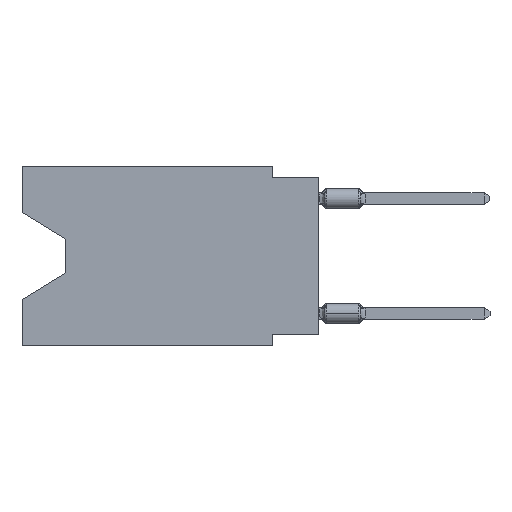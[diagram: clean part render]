
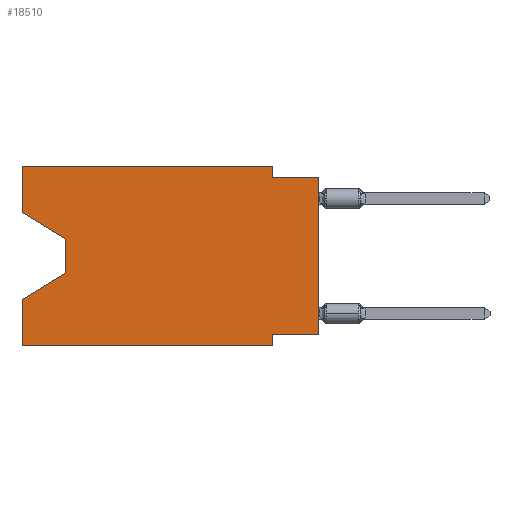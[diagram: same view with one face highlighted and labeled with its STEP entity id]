
A CAD part, left-side view. The second image highlights one B-rep face of the part: STEP entity #18510.
In plain terms, the highlighted planar face has unit normal (-1, 0, 0).
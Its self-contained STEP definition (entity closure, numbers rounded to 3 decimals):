
#665 = CARTESIAN_POINT ( 'NONE',  ( 0., 0., -0.635 ) ) ;
#674 = ORIENTED_EDGE ( 'NONE', *, *, #3548, .T. ) ;
#728 = LINE ( 'NONE', #2811, #1620 ) ;
#1167 = DIRECTION ( 'NONE',  ( 1., 0., 0. ) ) ;
#1458 = CARTESIAN_POINT ( 'NONE',  ( 0., 2.54, 0. ) ) ;
#1486 = ORIENTED_EDGE ( 'NONE', *, *, #24072, .F. ) ;
#1516 = VERTEX_POINT ( 'NONE', #9213 ) ;
#1619 = VERTEX_POINT ( 'NONE', #9345 ) ;
#1620 = VECTOR ( 'NONE', #18370, 1000. ) ;
#1637 = VERTEX_POINT ( 'NONE', #12419 ) ;
#2066 = VERTEX_POINT ( 'NONE', #665 ) ;
#2216 = VECTOR ( 'NONE', #14142, 1000. ) ;
#2474 = CARTESIAN_POINT ( 'NONE',  ( 0., 16.383, 0. ) ) ;
#2606 = VECTOR ( 'NONE', #7746, 1000. ) ;
#2622 = EDGE_CURVE ( 'NONE', #1619, #23544, #16702, .T. ) ;
#2811 = CARTESIAN_POINT ( 'NONE',  ( 0., 16.383, 0. ) ) ;
#2982 = AXIS2_PLACEMENT_3D ( 'NONE', #18926, #1167, #19428 ) ;
#3032 = VERTEX_POINT ( 'NONE', #24929 ) ;
#3123 = PLANE ( 'NONE',  #2982 ) ;
#3548 = EDGE_CURVE ( 'NONE', #1637, #2066, #16508, .T. ) ;
#4937 = CARTESIAN_POINT ( 'NONE',  ( 0., 16.383, -7.36 ) ) ;
#5001 = VECTOR ( 'NONE', #16237, 1000. ) ;
#5008 = VERTEX_POINT ( 'NONE', #15587 ) ;
#5181 = EDGE_CURVE ( 'NONE', #18726, #2066, #6169, .T. ) ;
#5586 = EDGE_LOOP ( 'NONE', ( #17032, #24458, #7455, #25322, #24687, #18570, #10149, #674, #22332, #18632, #1486, #10374 ) ) ;
#5853 = CARTESIAN_POINT ( 'NONE',  ( 0., 2.54, 0. ) ) ;
#5916 = VECTOR ( 'NONE', #11284, 1000. ) ;
#5964 = VECTOR ( 'NONE', #10813, 1000. ) ;
#5990 = DIRECTION ( 'NONE',  ( 0., 0., -1. ) ) ;
#6055 = LINE ( 'NONE', #19493, #2606 ) ;
#6169 = LINE ( 'NONE', #15846, #5001 ) ;
#6363 = VECTOR ( 'NONE', #22815, 1000. ) ;
#7059 = LINE ( 'NONE', #24748, #5964 ) ;
#7455 = ORIENTED_EDGE ( 'NONE', *, *, #19430, .T. ) ;
#7746 = DIRECTION ( 'NONE',  ( 0., -0.855, -0.519 ) ) ;
#8578 = EDGE_CURVE ( 'NONE', #25032, #18726, #14258, .T. ) ;
#8961 = CARTESIAN_POINT ( 'NONE',  ( 0., 16.383, 0. ) ) ;
#9213 = CARTESIAN_POINT ( 'NONE',  ( 0., 13.97, -5.893 ) ) ;
#9345 = CARTESIAN_POINT ( 'NONE',  ( 0., 16.383, -2.546 ) ) ;
#9884 = CARTESIAN_POINT ( 'NONE',  ( 0., 2.54, -0.635 ) ) ;
#9913 = CARTESIAN_POINT ( 'NONE',  ( 0., 13.97, -5.893 ) ) ;
#10149 = ORIENTED_EDGE ( 'NONE', *, *, #13811, .F. ) ;
#10374 = ORIENTED_EDGE ( 'NONE', *, *, #2622, .F. ) ;
#10813 = DIRECTION ( 'NONE',  ( 0., -1., 0. ) ) ;
#11152 = VECTOR ( 'NONE', #5990, 1000. ) ;
#11284 = DIRECTION ( 'NONE',  ( 0., 0., 1. ) ) ;
#11548 = VERTEX_POINT ( 'NONE', #15774 ) ;
#12119 = CARTESIAN_POINT ( 'NONE',  ( 0., 16.383, 0. ) ) ;
#12419 = CARTESIAN_POINT ( 'NONE',  ( 0., 0., -9.271 ) ) ;
#13000 = VECTOR ( 'NONE', #24486, 1000. ) ;
#13389 = VECTOR ( 'NONE', #21530, 1000. ) ;
#13648 = DIRECTION ( 'NONE',  ( 0., 0.855, -0.519 ) ) ;
#13811 = EDGE_CURVE ( 'NONE', #1637, #11548, #25047, .T. ) ;
#14142 = DIRECTION ( 'NONE',  ( 0., -1., 0. ) ) ;
#14258 = LINE ( 'NONE', #5853, #11152 ) ;
#14297 = LINE ( 'NONE', #22184, #13000 ) ;
#14510 = VERTEX_POINT ( 'NONE', #4937 ) ;
#14960 = DIRECTION ( 'NONE',  ( 0., 1., 0. ) ) ;
#15017 = VECTOR ( 'NONE', #13648, 1000. ) ;
#15587 = CARTESIAN_POINT ( 'NONE',  ( 0., 13.97, -4.013 ) ) ;
#15774 = CARTESIAN_POINT ( 'NONE',  ( 0., 2.54, -9.271 ) ) ;
#15846 = CARTESIAN_POINT ( 'NONE',  ( 0., 0., -0.635 ) ) ;
#16237 = DIRECTION ( 'NONE',  ( 0., -1., 0. ) ) ;
#16508 = LINE ( 'NONE', #24896, #13389 ) ;
#16702 = LINE ( 'NONE', #8961, #5916 ) ;
#17032 = ORIENTED_EDGE ( 'NONE', *, *, #18996, .T. ) ;
#17125 = VECTOR ( 'NONE', #14960, 1000. ) ;
#17431 = EDGE_CURVE ( 'NONE', #24689, #14510, #728, .T. ) ;
#17666 = LINE ( 'NONE', #9913, #15017 ) ;
#18370 = DIRECTION ( 'NONE',  ( 0., 0., 1. ) ) ;
#18413 = LINE ( 'NONE', #2474, #2216 ) ;
#18510 = ADVANCED_FACE ( 'NONE', ( #20850 ), #3123, .F. ) ;
#18570 = ORIENTED_EDGE ( 'NONE', *, *, #22584, .F. ) ;
#18632 = ORIENTED_EDGE ( 'NONE', *, *, #8578, .F. ) ;
#18726 = VERTEX_POINT ( 'NONE', #9884 ) ;
#18926 = CARTESIAN_POINT ( 'NONE',  ( 0., 16.383, 0. ) ) ;
#18996 = EDGE_CURVE ( 'NONE', #1619, #5008, #6055, .T. ) ;
#19209 = CARTESIAN_POINT ( 'NONE',  ( 0., 13.97, -4.013 ) ) ;
#19428 = DIRECTION ( 'NONE',  ( 0., 0., -1. ) ) ;
#19430 = EDGE_CURVE ( 'NONE', #1516, #14510, #17666, .T. ) ;
#19493 = CARTESIAN_POINT ( 'NONE',  ( 0., 16.383, -2.546 ) ) ;
#20850 = FACE_OUTER_BOUND ( 'NONE', #5586, .T. ) ;
#21530 = DIRECTION ( 'NONE',  ( 0., 0., 1. ) ) ;
#22184 = CARTESIAN_POINT ( 'NONE',  ( 0., 2.54, -9.906 ) ) ;
#22332 = ORIENTED_EDGE ( 'NONE', *, *, #5181, .F. ) ;
#22584 = EDGE_CURVE ( 'NONE', #11548, #3032, #14297, .T. ) ;
#22609 = EDGE_CURVE ( 'NONE', #24689, #3032, #7059, .T. ) ;
#22707 = CARTESIAN_POINT ( 'NONE',  ( 0., 0., -9.271 ) ) ;
#22815 = DIRECTION ( 'NONE',  ( 0., 0., -1. ) ) ;
#23070 = LINE ( 'NONE', #19209, #6363 ) ;
#23100 = CARTESIAN_POINT ( 'NONE',  ( 0., 16.383, -9.906 ) ) ;
#23544 = VERTEX_POINT ( 'NONE', #12119 ) ;
#24072 = EDGE_CURVE ( 'NONE', #23544, #25032, #18413, .T. ) ;
#24458 = ORIENTED_EDGE ( 'NONE', *, *, #25098, .T. ) ;
#24486 = DIRECTION ( 'NONE',  ( 0., 0., -1. ) ) ;
#24687 = ORIENTED_EDGE ( 'NONE', *, *, #22609, .T. ) ;
#24689 = VERTEX_POINT ( 'NONE', #23100 ) ;
#24748 = CARTESIAN_POINT ( 'NONE',  ( 0., 16.383, -9.906 ) ) ;
#24896 = CARTESIAN_POINT ( 'NONE',  ( 0., 0., 0. ) ) ;
#24929 = CARTESIAN_POINT ( 'NONE',  ( 0., 2.54, -9.906 ) ) ;
#25032 = VERTEX_POINT ( 'NONE', #1458 ) ;
#25047 = LINE ( 'NONE', #22707, #17125 ) ;
#25098 = EDGE_CURVE ( 'NONE', #5008, #1516, #23070, .T. ) ;
#25322 = ORIENTED_EDGE ( 'NONE', *, *, #17431, .F. ) ;
